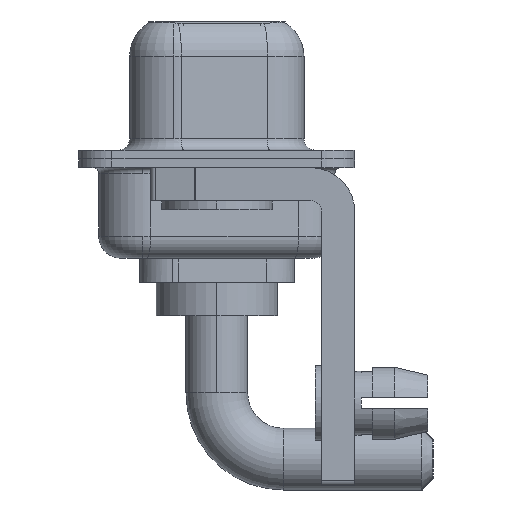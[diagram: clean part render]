
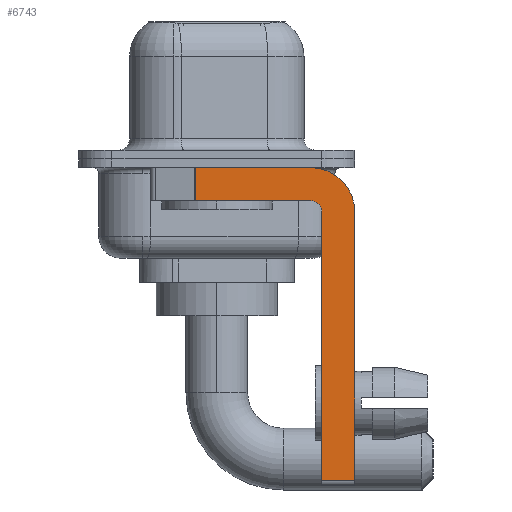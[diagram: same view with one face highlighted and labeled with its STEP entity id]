
A CAD part, left-side view. The second image highlights one B-rep face of the part: STEP entity #6743.
In plain terms, the highlighted planar face has unit normal (-1, 0, 0).
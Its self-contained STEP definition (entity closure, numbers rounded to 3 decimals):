
#97 = AXIS2_PLACEMENT_3D ( 'NONE', #12183, #3212, #5896 ) ;
#116 = EDGE_LOOP ( 'NONE', ( #10000, #14705, #14425, #13325, #9649, #7614, #7194, #7990 ) ) ;
#246 = EDGE_CURVE ( 'NONE', #3836, #15964, #12892, .T. ) ;
#326 = VERTEX_POINT ( 'NONE', #9683 ) ;
#551 = CARTESIAN_POINT ( 'NONE',  ( -2.9, -6.25, -2.4 ) ) ;
#991 = EDGE_CURVE ( 'NONE', #3829, #3280, #15131, .T. ) ;
#1053 = VERTEX_POINT ( 'NONE', #14880 ) ;
#1107 = LINE ( 'NONE', #13541, #15990 ) ;
#1120 = VECTOR ( 'NONE', #12327, 1000. ) ;
#1370 = DIRECTION ( 'NONE',  ( 0., -1., 0. ) ) ;
#2090 = LINE ( 'NONE', #9468, #5903 ) ;
#2387 = VERTEX_POINT ( 'NONE', #6088 ) ;
#2391 = CARTESIAN_POINT ( 'NONE',  ( -2.9, -4.75, -2.4 ) ) ;
#2594 = DIRECTION ( 'NONE',  ( 0., 0., -1. ) ) ;
#2698 = VECTOR ( 'NONE', #1370, 1000. ) ;
#2750 = PLANE ( 'NONE',  #11020 ) ;
#3071 = DIRECTION ( 'NONE',  ( 0., -1., 0. ) ) ;
#3212 = DIRECTION ( 'NONE',  ( -1., 0., 0. ) ) ;
#3280 = VERTEX_POINT ( 'NONE', #7876 ) ;
#3829 = VERTEX_POINT ( 'NONE', #16143 ) ;
#3836 = VERTEX_POINT ( 'NONE', #2391 ) ;
#4210 = DIRECTION ( 'NONE',  ( 1., 0., 0. ) ) ;
#4436 = CARTESIAN_POINT ( 'NONE',  ( -2.9, -6.25, -2.4 ) ) ;
#4606 = CARTESIAN_POINT ( 'NONE',  ( -2.9, 3., -0.4 ) ) ;
#5533 = DIRECTION ( 'NONE',  ( 0., 0., 1. ) ) ;
#5896 = DIRECTION ( 'NONE',  ( 0., 0., 1. ) ) ;
#5903 = VECTOR ( 'NONE', #5533, 1000. ) ;
#6088 = CARTESIAN_POINT ( 'NONE',  ( -2.9, -4.25, -0.4 ) ) ;
#6140 = EDGE_CURVE ( 'NONE', #3829, #3836, #2090, .T. ) ;
#6261 = EDGE_CURVE ( 'NONE', #1053, #326, #1107, .T. ) ;
#6743 = ADVANCED_FACE ( 'NONE', ( #14110 ), #2750, .F. ) ;
#6858 = CIRCLE ( 'NONE', #15242, 2. ) ;
#6870 = EDGE_CURVE ( 'NONE', #1053, #2387, #11956, .T. ) ;
#7194 = ORIENTED_EDGE ( 'NONE', *, *, #12221, .F. ) ;
#7417 = CARTESIAN_POINT ( 'NONE',  ( -2.9, -4.25, -14.55 ) ) ;
#7440 = DIRECTION ( 'NONE',  ( 0., 0., -1. ) ) ;
#7596 = EDGE_CURVE ( 'NONE', #15964, #326, #8519, .T. ) ;
#7614 = ORIENTED_EDGE ( 'NONE', *, *, #991, .T. ) ;
#7697 = VERTEX_POINT ( 'NONE', #551 ) ;
#7876 = CARTESIAN_POINT ( 'NONE',  ( -2.9, -6.25, -14.55 ) ) ;
#7990 = ORIENTED_EDGE ( 'NONE', *, *, #8903, .F. ) ;
#8120 = LINE ( 'NONE', #4436, #11328 ) ;
#8519 = LINE ( 'NONE', #8682, #1120 ) ;
#8682 = CARTESIAN_POINT ( 'NONE',  ( -2.9, -4.25, -1.9 ) ) ;
#8903 = EDGE_CURVE ( 'NONE', #2387, #7697, #6858, .T. ) ;
#9468 = CARTESIAN_POINT ( 'NONE',  ( -2.9, -4.75, -14.8 ) ) ;
#9649 = ORIENTED_EDGE ( 'NONE', *, *, #6140, .F. ) ;
#9683 = CARTESIAN_POINT ( 'NONE',  ( -2.9, 0.978, -1.9 ) ) ;
#9992 = DIRECTION ( 'NONE',  ( 1., 0., 0. ) ) ;
#10000 = ORIENTED_EDGE ( 'NONE', *, *, #6870, .F. ) ;
#11020 = AXIS2_PLACEMENT_3D ( 'NONE', #13861, #4210, #11404 ) ;
#11328 = VECTOR ( 'NONE', #15647, 1000. ) ;
#11404 = DIRECTION ( 'NONE',  ( 0., 0., -1. ) ) ;
#11956 = LINE ( 'NONE', #4606, #15482 ) ;
#12183 = CARTESIAN_POINT ( 'NONE',  ( -2.9, -4.25, -2.4 ) ) ;
#12221 = EDGE_CURVE ( 'NONE', #7697, #3280, #8120, .T. ) ;
#12298 = CARTESIAN_POINT ( 'NONE',  ( -2.9, -4.25, -1.9 ) ) ;
#12327 = DIRECTION ( 'NONE',  ( 0., 1., 0. ) ) ;
#12892 = CIRCLE ( 'NONE', #97, 0.5 ) ;
#13325 = ORIENTED_EDGE ( 'NONE', *, *, #246, .F. ) ;
#13541 = CARTESIAN_POINT ( 'NONE',  ( -2.9, 0.978, -1.9 ) ) ;
#13861 = CARTESIAN_POINT ( 'NONE',  ( -2.9, -4.25, -2.4 ) ) ;
#14110 = FACE_OUTER_BOUND ( 'NONE', #116, .T. ) ;
#14425 = ORIENTED_EDGE ( 'NONE', *, *, #7596, .F. ) ;
#14705 = ORIENTED_EDGE ( 'NONE', *, *, #6261, .T. ) ;
#14880 = CARTESIAN_POINT ( 'NONE',  ( -2.9, 0.978, -0.4 ) ) ;
#15131 = LINE ( 'NONE', #7417, #2698 ) ;
#15242 = AXIS2_PLACEMENT_3D ( 'NONE', #16124, #9992, #7440 ) ;
#15482 = VECTOR ( 'NONE', #3071, 1000. ) ;
#15647 = DIRECTION ( 'NONE',  ( 0., 0., -1. ) ) ;
#15964 = VERTEX_POINT ( 'NONE', #12298 ) ;
#15990 = VECTOR ( 'NONE', #2594, 1000. ) ;
#16124 = CARTESIAN_POINT ( 'NONE',  ( -2.9, -4.25, -2.4 ) ) ;
#16143 = CARTESIAN_POINT ( 'NONE',  ( -2.9, -4.75, -14.55 ) ) ;
